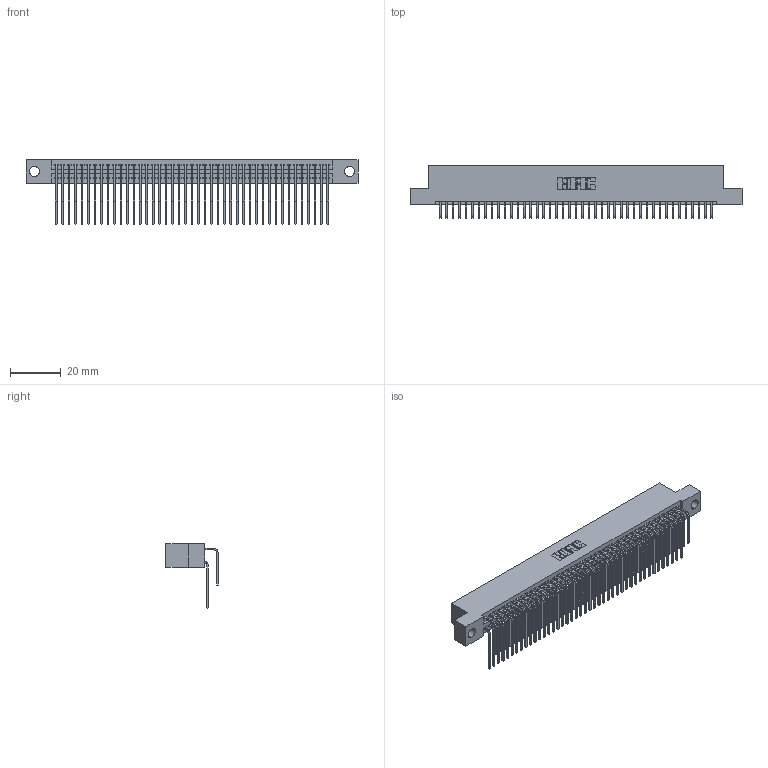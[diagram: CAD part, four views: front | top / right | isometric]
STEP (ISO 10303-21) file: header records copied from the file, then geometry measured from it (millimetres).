
FILE_DESCRIPTION (( 'STEP AP203' ), '1' );
FILE_NAME ('345-086-559-204.STEP', '2021-05-20T13:44:18', ( '' ), ( '' ), 'SwSTEP 2.0', 'SolidWorks 2020', '' );
FILE_SCHEMA (( 'CONFIG_CONTROL_DESIGN' ));
Length unit declared in the file: inch
Products named in the file (4): 345 Part_Flush Mounting Lugs - 0.156 Dia-TI; 345-086-559-204; 345-292-001_558 559 Tail - 1; 345-292-001_559 Tail - 2
Assembly tree (87 placements, depth 2):
  345-086-559-204
    345 Part_Flush Mounting Lugs - 0.156 Dia-TI
    345-292-001_558 559 Tail - 1  x43
    345-292-001_559 Tail - 2  x43
Bounding box: 130.43 x 20.56 x 25.53 mm (x, y, z)
Volume: 13069.4 mm3; surface area: 21522.7 mm2
Topology: 87 solids, 87 shells, 4612 faces, 13707 edges, 9022 vertices
Faces by surface type: plane 3104, cylinder 1508
Entity records: 35675 total; most frequent: CARTESIAN_POINT 6029, ORIENTED_EDGE 5910, DIRECTION 5287, EDGE_CURVE 2955, LINE 2611, VECTOR 2611, VERTEX_POINT 1966, AXIS2_PLACEMENT_3D 1338
